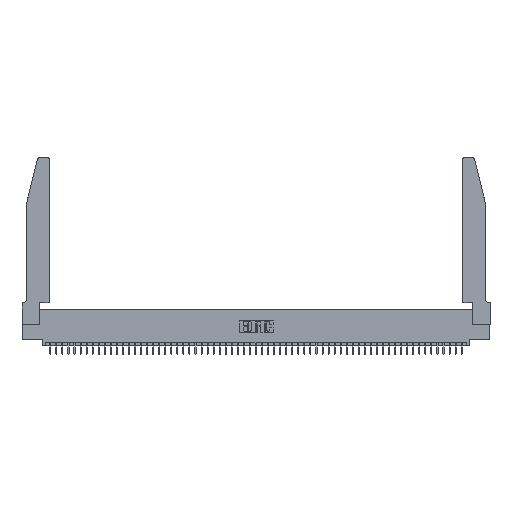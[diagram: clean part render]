
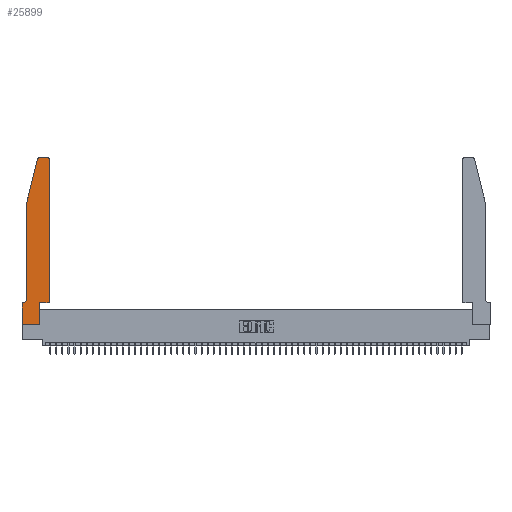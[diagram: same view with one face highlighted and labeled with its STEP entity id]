
A CAD part, top view. The second image highlights one B-rep face of the part: STEP entity #25899.
In plain terms, the highlighted planar face has unit normal (0, 0, 1).
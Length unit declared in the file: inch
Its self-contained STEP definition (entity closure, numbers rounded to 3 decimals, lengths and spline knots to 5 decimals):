
#134 = CARTESIAN_POINT ( 'NONE',  ( 0.2605, 2.75, 0.37 ) ) ;
#487 = FACE_OUTER_BOUND ( 'NONE', #33348, .T. ) ;
#797 = ORIENTED_EDGE ( 'NONE', *, *, #54308, .T. ) ;
#2430 = CARTESIAN_POINT ( 'NONE',  ( 0.2865, 0.35, 0.37 ) ) ;
#2456 = VERTEX_POINT ( 'NONE', #51490 ) ;
#3322 = EDGE_CURVE ( 'NONE', #20263, #31801, #26052, .T. ) ;
#3936 = CIRCLE ( 'NONE', #21891, 0.07 ) ;
#4371 = EDGE_CURVE ( 'NONE', #24990, #2456, #27784, .T. ) ;
#4708 = VECTOR ( 'NONE', #31425, 39.37008 ) ;
#4886 = EDGE_CURVE ( 'NONE', #23623, #42920, #31931, .T. ) ;
#5968 = DIRECTION ( 'NONE',  ( 1., 0., 0. ) ) ;
#6694 = CARTESIAN_POINT ( 'NONE',  ( 0., 0., 0.37 ) ) ;
#6798 = VECTOR ( 'NONE', #21749, 39.37008 ) ;
#6909 = LINE ( 'NONE', #20947, #36923 ) ;
#6957 = CIRCLE ( 'NONE', #48245, 0.03 ) ;
#7395 = CARTESIAN_POINT ( 'NONE',  ( 0.0755, 0.35, 0.37 ) ) ;
#7709 = CARTESIAN_POINT ( 'NONE',  ( 0., 0.35, 0.37 ) ) ;
#7736 = ORIENTED_EDGE ( 'NONE', *, *, #37990, .T. ) ;
#8403 = VERTEX_POINT ( 'NONE', #44213 ) ;
#10649 = CARTESIAN_POINT ( 'NONE',  ( 0.0755, 2., 0.37 ) ) ;
#11282 = CARTESIAN_POINT ( 'NONE',  ( 0.284, 2.72, 0.37 ) ) ;
#11479 = VERTEX_POINT ( 'NONE', #16938 ) ;
#11620 = LINE ( 'NONE', #7395, #24486 ) ;
#13216 = VERTEX_POINT ( 'NONE', #13221 ) ;
#13221 = CARTESIAN_POINT ( 'NONE',  ( 0.0055, 0.35, 0.37 ) ) ;
#14889 = DIRECTION ( 'NONE',  ( -1., 0., 0. ) ) ;
#15360 = DIRECTION ( 'NONE',  ( 1., 0., 0. ) ) ;
#15839 = CARTESIAN_POINT ( 'NONE',  ( 0.0755, 0.42, 0.37 ) ) ;
#16635 = EDGE_CURVE ( 'NONE', #39012, #33657, #38055, .T. ) ;
#16938 = CARTESIAN_POINT ( 'NONE',  ( 0.4505, 2.72, 0.37 ) ) ;
#17904 = DIRECTION ( 'NONE',  ( 0., 0., 1. ) ) ;
#17914 = CARTESIAN_POINT ( 'NONE',  ( 0., 0., 0.37 ) ) ;
#18003 = ORIENTED_EDGE ( 'NONE', *, *, #55208, .T. ) ;
#18203 = CARTESIAN_POINT ( 'NONE',  ( 0.25487, 2.72718, 0.37 ) ) ;
#18649 = ORIENTED_EDGE ( 'NONE', *, *, #3322, .T. ) ;
#19121 = DIRECTION ( 'NONE',  ( 0., 0., -1. ) ) ;
#19194 = ORIENTED_EDGE ( 'NONE', *, *, #21898, .T. ) ;
#20263 = VERTEX_POINT ( 'NONE', #7709 ) ;
#20947 = CARTESIAN_POINT ( 'NONE',  ( 0.0755, 2., 0.37 ) ) ;
#21474 = LINE ( 'NONE', #29889, #30790 ) ;
#21749 = DIRECTION ( 'NONE',  ( -1., 0., 0. ) ) ;
#21891 = AXIS2_PLACEMENT_3D ( 'NONE', #27548, #19121, #14889 ) ;
#21898 = EDGE_CURVE ( 'NONE', #42920, #8403, #53517, .T. ) ;
#22580 = ORIENTED_EDGE ( 'NONE', *, *, #16635, .T. ) ;
#23623 = VERTEX_POINT ( 'NONE', #43412 ) ;
#24373 = CIRCLE ( 'NONE', #31550, 0.03 ) ;
#24486 = VECTOR ( 'NONE', #37451, 39.37008 ) ;
#24990 = VERTEX_POINT ( 'NONE', #18203 ) ;
#25543 = ORIENTED_EDGE ( 'NONE', *, *, #36394, .T. ) ;
#25770 = CARTESIAN_POINT ( 'NONE',  ( 0., 0.35, 0.37 ) ) ;
#25899 = ADVANCED_FACE ( 'NONE', ( #487 ), #26320, .T. ) ;
#26052 = LINE ( 'NONE', #17914, #37817 ) ;
#26320 = PLANE ( 'NONE',  #30473 ) ;
#26604 = DIRECTION ( 'NONE',  ( 0., -1., 0. ) ) ;
#27548 = CARTESIAN_POINT ( 'NONE',  ( 0.0055, 0.42, 0.37 ) ) ;
#27784 = LINE ( 'NONE', #10649, #4708 ) ;
#28006 = LINE ( 'NONE', #49094, #28365 ) ;
#28365 = VECTOR ( 'NONE', #15360, 39.37008 ) ;
#29889 = CARTESIAN_POINT ( 'NONE',  ( 0.4505, 0.35, 0.37 ) ) ;
#30473 = AXIS2_PLACEMENT_3D ( 'NONE', #25770, #17904, #43747 ) ;
#30790 = VECTOR ( 'NONE', #47326, 39.37008 ) ;
#31425 = DIRECTION ( 'NONE',  ( -0.239, -0.971, 0. ) ) ;
#31550 = AXIS2_PLACEMENT_3D ( 'NONE', #11282, #32072, #5968 ) ;
#31801 = VERTEX_POINT ( 'NONE', #6694 ) ;
#31825 = ORIENTED_EDGE ( 'NONE', *, *, #50687, .T. ) ;
#31931 = LINE ( 'NONE', #36429, #48891 ) ;
#32072 = DIRECTION ( 'NONE',  ( 0., 0., 1. ) ) ;
#32690 = DIRECTION ( 'NONE',  ( 1., 0., 0. ) ) ;
#33348 = EDGE_LOOP ( 'NONE', ( #22580, #31825, #44315, #25543, #18003, #7736, #18649, #40434, #51954, #19194, #797, #53012 ) ) ;
#33657 = VERTEX_POINT ( 'NONE', #54678 ) ;
#36394 = EDGE_CURVE ( 'NONE', #2456, #44548, #6909, .T. ) ;
#36429 = CARTESIAN_POINT ( 'NONE',  ( 0.2865, 0.35, 0.37 ) ) ;
#36640 = CARTESIAN_POINT ( 'NONE',  ( 0.4205, 2.75, 0.37 ) ) ;
#36913 = CARTESIAN_POINT ( 'NONE',  ( 0.4505, 0.35, 0.37 ) ) ;
#36923 = VECTOR ( 'NONE', #50158, 39.37008 ) ;
#37451 = DIRECTION ( 'NONE',  ( -1., 0., 0. ) ) ;
#37817 = VECTOR ( 'NONE', #26604, 39.37008 ) ;
#37990 = EDGE_CURVE ( 'NONE', #13216, #20263, #11620, .T. ) ;
#38055 = LINE ( 'NONE', #134, #6798 ) ;
#39012 = VERTEX_POINT ( 'NONE', #36640 ) ;
#40434 = ORIENTED_EDGE ( 'NONE', *, *, #45938, .T. ) ;
#41108 = VECTOR ( 'NONE', #32690, 39.37008 ) ;
#42920 = VERTEX_POINT ( 'NONE', #2430 ) ;
#43011 = DIRECTION ( 'NONE',  ( 0., 0., 1. ) ) ;
#43412 = CARTESIAN_POINT ( 'NONE',  ( 0.2865, 0., 0.37 ) ) ;
#43747 = DIRECTION ( 'NONE',  ( 1., 0., 0. ) ) ;
#44213 = CARTESIAN_POINT ( 'NONE',  ( 0.4505, 0.35, 0.37 ) ) ;
#44315 = ORIENTED_EDGE ( 'NONE', *, *, #4371, .T. ) ;
#44548 = VERTEX_POINT ( 'NONE', #15839 ) ;
#45195 = EDGE_CURVE ( 'NONE', #11479, #39012, #6957, .T. ) ;
#45938 = EDGE_CURVE ( 'NONE', #31801, #23623, #28006, .T. ) ;
#46412 = DIRECTION ( 'NONE',  ( 1., 0., 0. ) ) ;
#47326 = DIRECTION ( 'NONE',  ( 0., 1., 0. ) ) ;
#48245 = AXIS2_PLACEMENT_3D ( 'NONE', #55399, #43011, #46412 ) ;
#48891 = VECTOR ( 'NONE', #49350, 39.37008 ) ;
#49094 = CARTESIAN_POINT ( 'NONE',  ( 0., 0., 0.37 ) ) ;
#49350 = DIRECTION ( 'NONE',  ( 0., 1., 0. ) ) ;
#50158 = DIRECTION ( 'NONE',  ( 0., -1., 0. ) ) ;
#50687 = EDGE_CURVE ( 'NONE', #33657, #24990, #24373, .T. ) ;
#51490 = CARTESIAN_POINT ( 'NONE',  ( 0.0755, 2., 0.37 ) ) ;
#51954 = ORIENTED_EDGE ( 'NONE', *, *, #4886, .T. ) ;
#53012 = ORIENTED_EDGE ( 'NONE', *, *, #45195, .T. ) ;
#53517 = LINE ( 'NONE', #36913, #41108 ) ;
#54308 = EDGE_CURVE ( 'NONE', #8403, #11479, #21474, .T. ) ;
#54678 = CARTESIAN_POINT ( 'NONE',  ( 0.284, 2.75, 0.37 ) ) ;
#55208 = EDGE_CURVE ( 'NONE', #44548, #13216, #3936, .T. ) ;
#55399 = CARTESIAN_POINT ( 'NONE',  ( 0.4205, 2.72, 0.37 ) ) ;
